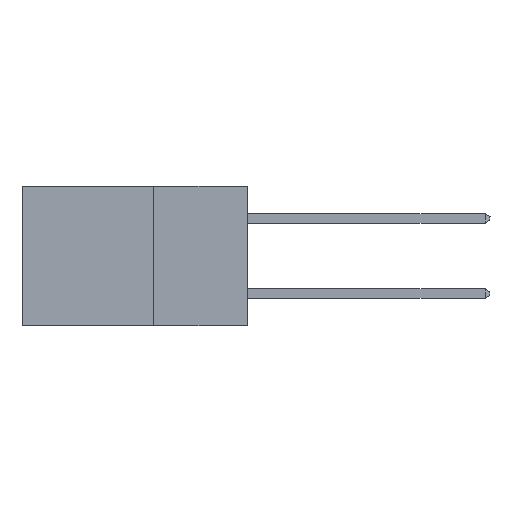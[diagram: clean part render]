
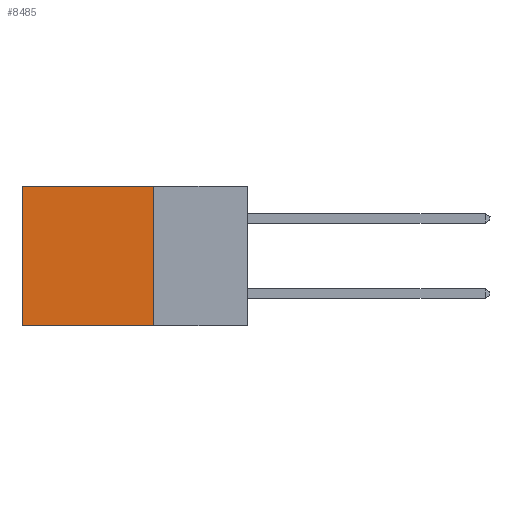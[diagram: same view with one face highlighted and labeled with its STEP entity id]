
A CAD part, left-side view. The second image highlights one B-rep face of the part: STEP entity #8485.
In plain terms, the highlighted planar face has unit normal (-1, 0, 0).
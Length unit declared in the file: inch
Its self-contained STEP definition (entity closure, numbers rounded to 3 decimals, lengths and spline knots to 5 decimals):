
#994 = DIRECTION ( 'NONE',  ( 0., 0., -1. ) ) ;
#1658 = CARTESIAN_POINT ( 'NONE',  ( 0.298, 0.6, 0. ) ) ;
#1726 = VERTEX_POINT ( 'NONE', #6550 ) ;
#1924 = LINE ( 'NONE', #14754, #4921 ) ;
#3737 = DIRECTION ( 'NONE',  ( 0., 0., -1. ) ) ;
#4921 = VECTOR ( 'NONE', #7480, 39.37008 ) ;
#5508 = LINE ( 'NONE', #13170, #14419 ) ;
#6550 = CARTESIAN_POINT ( 'NONE',  ( 0.298, 0.25, 0. ) ) ;
#7127 = CARTESIAN_POINT ( 'NONE',  ( 0.298, 0.25, -0.37 ) ) ;
#7480 = DIRECTION ( 'NONE',  ( 0., 1., 0. ) ) ;
#7914 = EDGE_LOOP ( 'NONE', ( #9425, #29107, #9515, #20137 ) ) ;
#8168 = CARTESIAN_POINT ( 'NONE',  ( 0.298, 0.25, -0.37 ) ) ;
#8485 = ADVANCED_FACE ( 'NONE', ( #25361 ), #22295, .F. ) ;
#9425 = ORIENTED_EDGE ( 'NONE', *, *, #28645, .T. ) ;
#9515 = ORIENTED_EDGE ( 'NONE', *, *, #12672, .F. ) ;
#9562 = EDGE_CURVE ( 'NONE', #1726, #28230, #1924, .T. ) ;
#9747 = AXIS2_PLACEMENT_3D ( 'NONE', #22185, #27016, #994 ) ;
#10133 = EDGE_CURVE ( 'NONE', #17796, #16380, #23776, .T. ) ;
#12672 = EDGE_CURVE ( 'NONE', #1726, #17796, #5508, .T. ) ;
#13170 = CARTESIAN_POINT ( 'NONE',  ( 0.298, 0.25, 0. ) ) ;
#14419 = VECTOR ( 'NONE', #3737, 39.37008 ) ;
#14754 = CARTESIAN_POINT ( 'NONE',  ( 0.298, 0.25, 0. ) ) ;
#16380 = VERTEX_POINT ( 'NONE', #21959 ) ;
#17796 = VERTEX_POINT ( 'NONE', #7127 ) ;
#20137 = ORIENTED_EDGE ( 'NONE', *, *, #9562, .T. ) ;
#21959 = CARTESIAN_POINT ( 'NONE',  ( 0.298, 0.6, -0.37 ) ) ;
#22185 = CARTESIAN_POINT ( 'NONE',  ( 0.298, 0.25, 0. ) ) ;
#22295 = PLANE ( 'NONE',  #9747 ) ;
#22613 = VECTOR ( 'NONE', #23408, 39.37008 ) ;
#22685 = VECTOR ( 'NONE', #27293, 39.37008 ) ;
#23312 = LINE ( 'NONE', #1658, #22613 ) ;
#23408 = DIRECTION ( 'NONE',  ( 0., 0., -1. ) ) ;
#23776 = LINE ( 'NONE', #8168, #22685 ) ;
#25361 = FACE_OUTER_BOUND ( 'NONE', #7914, .T. ) ;
#27016 = DIRECTION ( 'NONE',  ( 1., 0., 0. ) ) ;
#27293 = DIRECTION ( 'NONE',  ( 0., 1., 0. ) ) ;
#27714 = CARTESIAN_POINT ( 'NONE',  ( 0.298, 0.6, 0. ) ) ;
#28230 = VERTEX_POINT ( 'NONE', #27714 ) ;
#28645 = EDGE_CURVE ( 'NONE', #28230, #16380, #23312, .T. ) ;
#29107 = ORIENTED_EDGE ( 'NONE', *, *, #10133, .F. ) ;
